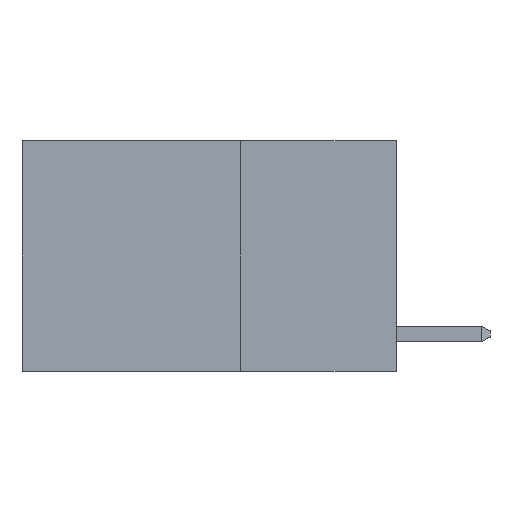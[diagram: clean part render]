
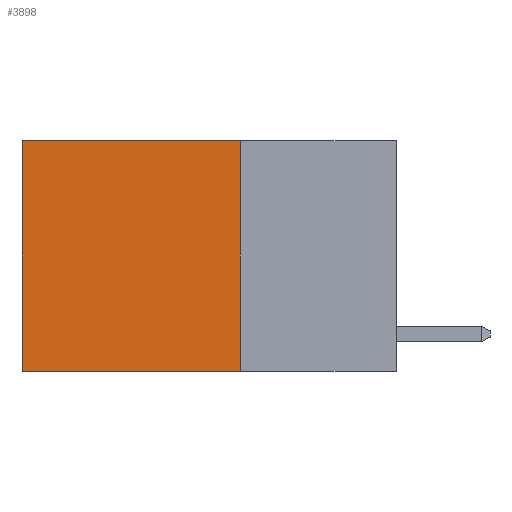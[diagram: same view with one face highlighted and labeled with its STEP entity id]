
A CAD part, left-side view. The second image highlights one B-rep face of the part: STEP entity #3898.
In plain terms, the highlighted planar face has unit normal (-1, 0, 0).
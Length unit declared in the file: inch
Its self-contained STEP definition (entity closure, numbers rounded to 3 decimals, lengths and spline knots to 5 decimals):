
#980 = LINE ( 'NONE', #1994, #6663 ) ;
#1469 = VERTEX_POINT ( 'NONE', #7708 ) ;
#1501 = VERTEX_POINT ( 'NONE', #6333 ) ;
#1994 = CARTESIAN_POINT ( 'NONE',  ( 0.2625, 0.25, -0.37 ) ) ;
#2173 = DIRECTION ( 'NONE',  ( 0., 1., 0. ) ) ;
#2209 = AXIS2_PLACEMENT_3D ( 'NONE', #4542, #8770, #4575 ) ;
#2280 = VECTOR ( 'NONE', #8835, 39.37008 ) ;
#2363 = ORIENTED_EDGE ( 'NONE', *, *, #9085, .F. ) ;
#2476 = EDGE_CURVE ( 'NONE', #1469, #1501, #6342, .T. ) ;
#2774 = ORIENTED_EDGE ( 'NONE', *, *, #2476, .T. ) ;
#3315 = ORIENTED_EDGE ( 'NONE', *, *, #4250, .F. ) ;
#3696 = ORIENTED_EDGE ( 'NONE', *, *, #5755, .T. ) ;
#3729 = LINE ( 'NONE', #6573, #7287 ) ;
#3898 = ADVANCED_FACE ( 'NONE', ( #4113 ), #7380, .F. ) ;
#4113 = FACE_OUTER_BOUND ( 'NONE', #5021, .T. ) ;
#4250 = EDGE_CURVE ( 'NONE', #9563, #1501, #980, .T. ) ;
#4542 = CARTESIAN_POINT ( 'NONE',  ( 0.2625, 0.25, 0. ) ) ;
#4575 = DIRECTION ( 'NONE',  ( 0., 0., -1. ) ) ;
#5021 = EDGE_LOOP ( 'NONE', ( #2774, #3315, #2363, #3696 ) ) ;
#5442 = DIRECTION ( 'NONE',  ( 0., 0., -1. ) ) ;
#5755 = EDGE_CURVE ( 'NONE', #8251, #1469, #3729, .T. ) ;
#6055 = CARTESIAN_POINT ( 'NONE',  ( 0.2625, 0.25, 0. ) ) ;
#6140 = VECTOR ( 'NONE', #5442, 39.37008 ) ;
#6333 = CARTESIAN_POINT ( 'NONE',  ( 0.2625, 0.6, -0.37 ) ) ;
#6342 = LINE ( 'NONE', #7506, #6140 ) ;
#6573 = CARTESIAN_POINT ( 'NONE',  ( 0.2625, 0.25, 0. ) ) ;
#6663 = VECTOR ( 'NONE', #7786, 39.37008 ) ;
#7287 = VECTOR ( 'NONE', #2173, 39.37008 ) ;
#7380 = PLANE ( 'NONE',  #2209 ) ;
#7506 = CARTESIAN_POINT ( 'NONE',  ( 0.2625, 0.6, 0. ) ) ;
#7708 = CARTESIAN_POINT ( 'NONE',  ( 0.2625, 0.6, 0. ) ) ;
#7786 = DIRECTION ( 'NONE',  ( 0., 1., 0. ) ) ;
#8036 = LINE ( 'NONE', #6055, #2280 ) ;
#8251 = VERTEX_POINT ( 'NONE', #9452 ) ;
#8631 = CARTESIAN_POINT ( 'NONE',  ( 0.2625, 0.25, -0.37 ) ) ;
#8770 = DIRECTION ( 'NONE',  ( 1., 0., 0. ) ) ;
#8835 = DIRECTION ( 'NONE',  ( 0., 0., -1. ) ) ;
#9085 = EDGE_CURVE ( 'NONE', #8251, #9563, #8036, .T. ) ;
#9452 = CARTESIAN_POINT ( 'NONE',  ( 0.2625, 0.25, 0. ) ) ;
#9563 = VERTEX_POINT ( 'NONE', #8631 ) ;
